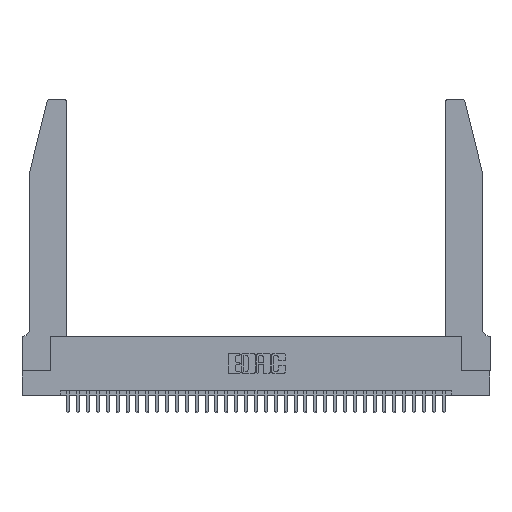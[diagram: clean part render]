
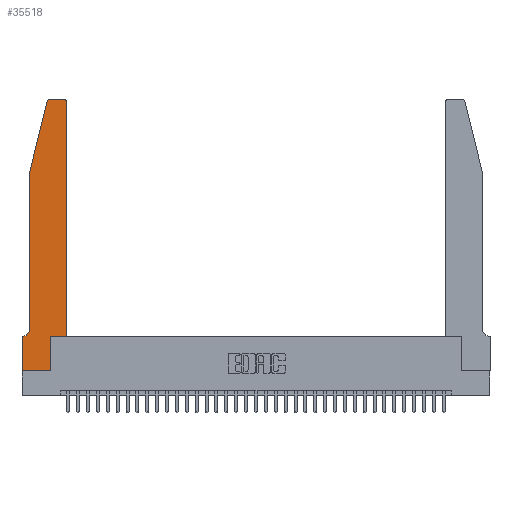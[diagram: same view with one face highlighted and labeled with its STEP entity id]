
A CAD part, top view. The second image highlights one B-rep face of the part: STEP entity #35518.
In plain terms, the highlighted planar face has unit normal (0, 0, 1).
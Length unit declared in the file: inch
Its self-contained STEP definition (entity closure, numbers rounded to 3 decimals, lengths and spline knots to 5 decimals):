
#701 = VERTEX_POINT ( 'NONE', #29468 ) ;
#905 = CARTESIAN_POINT ( 'NONE',  ( 0., 0., 0.37 ) ) ;
#953 = ORIENTED_EDGE ( 'NONE', *, *, #20223, .T. ) ;
#2262 = ORIENTED_EDGE ( 'NONE', *, *, #4411, .T. ) ;
#2562 = CIRCLE ( 'NONE', #5107, 0.03 ) ;
#2615 = LINE ( 'NONE', #16064, #9301 ) ;
#3031 = CARTESIAN_POINT ( 'NONE',  ( 0., 0.35, 0.37 ) ) ;
#3061 = VERTEX_POINT ( 'NONE', #12204 ) ;
#3322 = CARTESIAN_POINT ( 'NONE',  ( 0.0055, 0.35, 0.37 ) ) ;
#3348 = EDGE_CURVE ( 'NONE', #32725, #27830, #35198, .T. ) ;
#3352 = CARTESIAN_POINT ( 'NONE',  ( 0.2865, 0., 0.37 ) ) ;
#3651 = EDGE_CURVE ( 'NONE', #28948, #12194, #26719, .T. ) ;
#3701 = ORIENTED_EDGE ( 'NONE', *, *, #14805, .T. ) ;
#3839 = CARTESIAN_POINT ( 'NONE',  ( 0.0755, 0.35, 0.37 ) ) ;
#4078 = CARTESIAN_POINT ( 'NONE',  ( 0.4205, 2.72, 0.37 ) ) ;
#4411 = EDGE_CURVE ( 'NONE', #27830, #701, #10645, .T. ) ;
#4450 = CARTESIAN_POINT ( 'NONE',  ( 0.4505, 0.35, 0.37 ) ) ;
#4730 = CARTESIAN_POINT ( 'NONE',  ( 0.2865, 0.35, 0.37 ) ) ;
#4846 = VECTOR ( 'NONE', #13252, 39.37008 ) ;
#5081 = DIRECTION ( 'NONE',  ( -1., 0., 0. ) ) ;
#5107 = AXIS2_PLACEMENT_3D ( 'NONE', #4078, #23612, #6935 ) ;
#5143 = EDGE_CURVE ( 'NONE', #701, #34807, #2615, .T. ) ;
#5204 = VECTOR ( 'NONE', #28788, 39.37008 ) ;
#5513 = CARTESIAN_POINT ( 'NONE',  ( 0.2865, 0.35, 0.37 ) ) ;
#6606 = ORIENTED_EDGE ( 'NONE', *, *, #11167, .T. ) ;
#6935 = DIRECTION ( 'NONE',  ( 1., 0., 0. ) ) ;
#7448 = CARTESIAN_POINT ( 'NONE',  ( 0.25487, 2.72718, 0.37 ) ) ;
#7581 = DIRECTION ( 'NONE',  ( 0., 1., 0. ) ) ;
#7994 = CARTESIAN_POINT ( 'NONE',  ( 0.4505, 2.72, 0.37 ) ) ;
#8070 = VERTEX_POINT ( 'NONE', #7994 ) ;
#8101 = DIRECTION ( 'NONE',  ( 0., 0., 1. ) ) ;
#8750 = PLANE ( 'NONE',  #10700 ) ;
#9301 = VECTOR ( 'NONE', #35174, 39.37008 ) ;
#10026 = VECTOR ( 'NONE', #30368, 39.37008 ) ;
#10424 = CARTESIAN_POINT ( 'NONE',  ( 0.4505, 0.35, 0.37 ) ) ;
#10429 = CARTESIAN_POINT ( 'NONE',  ( 0.0055, 0.42, 0.37 ) ) ;
#10645 = LINE ( 'NONE', #21213, #31749 ) ;
#10700 = AXIS2_PLACEMENT_3D ( 'NONE', #3031, #11572, #30826 ) ;
#10962 = CARTESIAN_POINT ( 'NONE',  ( 0., 0.35, 0.37 ) ) ;
#10988 = VECTOR ( 'NONE', #7581, 39.37008 ) ;
#11167 = EDGE_CURVE ( 'NONE', #34807, #21962, #34223, .T. ) ;
#11572 = DIRECTION ( 'NONE',  ( 0., 0., 1. ) ) ;
#12036 = VECTOR ( 'NONE', #17629, 39.37008 ) ;
#12194 = VERTEX_POINT ( 'NONE', #4450 ) ;
#12204 = CARTESIAN_POINT ( 'NONE',  ( 0.4205, 2.75, 0.37 ) ) ;
#12479 = ORIENTED_EDGE ( 'NONE', *, *, #26404, .T. ) ;
#13252 = DIRECTION ( 'NONE',  ( 0., 1., 0. ) ) ;
#13254 = DIRECTION ( 'NONE',  ( -1., 0., 0. ) ) ;
#13718 = VERTEX_POINT ( 'NONE', #3352 ) ;
#13939 = LINE ( 'NONE', #21818, #28573 ) ;
#13965 = ORIENTED_EDGE ( 'NONE', *, *, #3651, .T. ) ;
#14805 = EDGE_CURVE ( 'NONE', #35872, #13718, #24758, .T. ) ;
#16064 = CARTESIAN_POINT ( 'NONE',  ( 0.0755, 2., 0.37 ) ) ;
#16858 = CARTESIAN_POINT ( 'NONE',  ( 0.0755, 0.42, 0.37 ) ) ;
#17181 = ORIENTED_EDGE ( 'NONE', *, *, #21681, .T. ) ;
#17629 = DIRECTION ( 'NONE',  ( 1., 0., 0. ) ) ;
#17646 = ORIENTED_EDGE ( 'NONE', *, *, #3348, .T. ) ;
#20223 = EDGE_CURVE ( 'NONE', #8070, #3061, #2562, .T. ) ;
#21213 = CARTESIAN_POINT ( 'NONE',  ( 0.0755, 2., 0.37 ) ) ;
#21681 = EDGE_CURVE ( 'NONE', #3061, #32725, #13939, .T. ) ;
#21818 = CARTESIAN_POINT ( 'NONE',  ( 0.2605, 2.75, 0.37 ) ) ;
#21962 = VERTEX_POINT ( 'NONE', #3322 ) ;
#21978 = VECTOR ( 'NONE', #26157, 39.37008 ) ;
#22707 = AXIS2_PLACEMENT_3D ( 'NONE', #10429, #29720, #13254 ) ;
#23612 = DIRECTION ( 'NONE',  ( 0., 0., 1. ) ) ;
#23978 = DIRECTION ( 'NONE',  ( -0.239, -0.971, 0. ) ) ;
#24756 = CARTESIAN_POINT ( 'NONE',  ( 0.284, 2.72, 0.37 ) ) ;
#24758 = LINE ( 'NONE', #33110, #10026 ) ;
#25960 = EDGE_CURVE ( 'NONE', #13718, #28948, #27053, .T. ) ;
#26157 = DIRECTION ( 'NONE',  ( -1., 0., 0. ) ) ;
#26404 = EDGE_CURVE ( 'NONE', #21962, #28892, #28395, .T. ) ;
#26425 = CARTESIAN_POINT ( 'NONE',  ( 0.284, 2.75, 0.37 ) ) ;
#26577 = LINE ( 'NONE', #10424, #10988 ) ;
#26719 = LINE ( 'NONE', #31267, #12036 ) ;
#27053 = LINE ( 'NONE', #4730, #4846 ) ;
#27389 = LINE ( 'NONE', #905, #5204 ) ;
#27486 = DIRECTION ( 'NONE',  ( 1., 0., 0. ) ) ;
#27830 = VERTEX_POINT ( 'NONE', #7448 ) ;
#28190 = ORIENTED_EDGE ( 'NONE', *, *, #25960, .T. ) ;
#28395 = LINE ( 'NONE', #3839, #21978 ) ;
#28573 = VECTOR ( 'NONE', #5081, 39.37008 ) ;
#28788 = DIRECTION ( 'NONE',  ( 0., -1., 0. ) ) ;
#28892 = VERTEX_POINT ( 'NONE', #10962 ) ;
#28948 = VERTEX_POINT ( 'NONE', #5513 ) ;
#29135 = ORIENTED_EDGE ( 'NONE', *, *, #32910, .T. ) ;
#29188 = ORIENTED_EDGE ( 'NONE', *, *, #5143, .T. ) ;
#29211 = EDGE_CURVE ( 'NONE', #28892, #35872, #27389, .T. ) ;
#29468 = CARTESIAN_POINT ( 'NONE',  ( 0.0755, 2., 0.37 ) ) ;
#29720 = DIRECTION ( 'NONE',  ( 0., 0., -1. ) ) ;
#30368 = DIRECTION ( 'NONE',  ( 1., 0., 0. ) ) ;
#30718 = EDGE_LOOP ( 'NONE', ( #17181, #17646, #2262, #29188, #6606, #12479, #34787, #3701, #28190, #13965, #29135, #953 ) ) ;
#30826 = DIRECTION ( 'NONE',  ( 1., 0., 0. ) ) ;
#31267 = CARTESIAN_POINT ( 'NONE',  ( 0.4505, 0.35, 0.37 ) ) ;
#31749 = VECTOR ( 'NONE', #23978, 39.37008 ) ;
#32103 = CARTESIAN_POINT ( 'NONE',  ( 0., 0., 0.37 ) ) ;
#32725 = VERTEX_POINT ( 'NONE', #26425 ) ;
#32910 = EDGE_CURVE ( 'NONE', #12194, #8070, #26577, .T. ) ;
#33110 = CARTESIAN_POINT ( 'NONE',  ( 0., 0., 0.37 ) ) ;
#33277 = AXIS2_PLACEMENT_3D ( 'NONE', #24756, #8101, #27486 ) ;
#34223 = CIRCLE ( 'NONE', #22707, 0.07 ) ;
#34787 = ORIENTED_EDGE ( 'NONE', *, *, #29211, .T. ) ;
#34807 = VERTEX_POINT ( 'NONE', #16858 ) ;
#35174 = DIRECTION ( 'NONE',  ( 0., -1., 0. ) ) ;
#35198 = CIRCLE ( 'NONE', #33277, 0.03 ) ;
#35249 = FACE_OUTER_BOUND ( 'NONE', #30718, .T. ) ;
#35518 = ADVANCED_FACE ( 'NONE', ( #35249 ), #8750, .T. ) ;
#35872 = VERTEX_POINT ( 'NONE', #32103 ) ;
